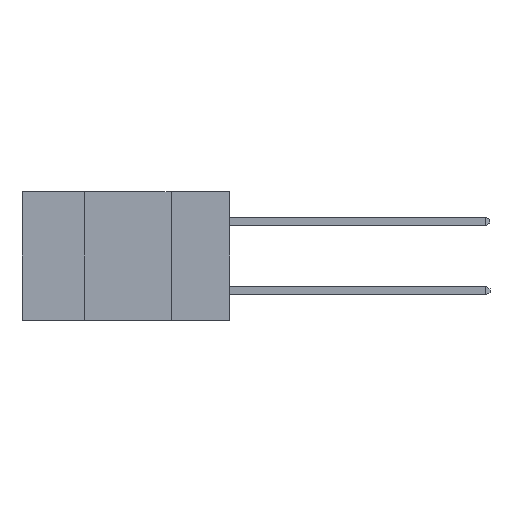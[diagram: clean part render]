
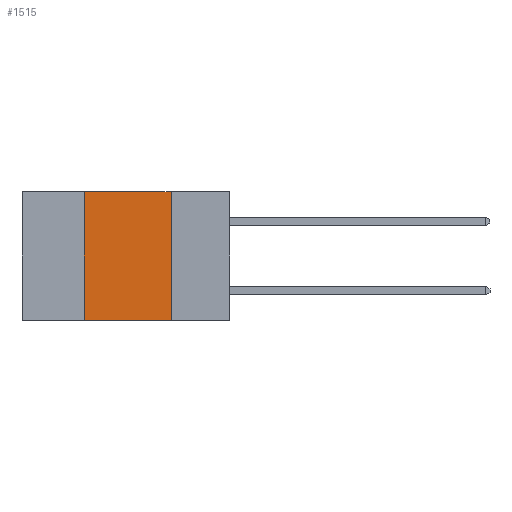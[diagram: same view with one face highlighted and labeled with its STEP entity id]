
A CAD part, left-side view. The second image highlights one B-rep face of the part: STEP entity #1515.
In plain terms, the highlighted planar face has unit normal (-1, 0, 0).
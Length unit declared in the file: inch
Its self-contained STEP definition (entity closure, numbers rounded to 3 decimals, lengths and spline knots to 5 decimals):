
#405 = VECTOR ( 'NONE', #3764, 39.37008 ) ;
#472 = CARTESIAN_POINT ( 'NONE',  ( 0., 0.6, 0. ) ) ;
#948 = LINE ( 'NONE', #8181, #2909 ) ;
#1068 = ORIENTED_EDGE ( 'NONE', *, *, #5798, .T. ) ;
#1515 = ADVANCED_FACE ( 'NONE', ( #8056 ), #9305, .F. ) ;
#2367 = CARTESIAN_POINT ( 'NONE',  ( 0., 0.42, 0. ) ) ;
#2909 = VECTOR ( 'NONE', #7818, 39.37008 ) ;
#3309 = CARTESIAN_POINT ( 'NONE',  ( 0., 0.42, -0.37 ) ) ;
#3413 = VERTEX_POINT ( 'NONE', #5740 ) ;
#3545 = ORIENTED_EDGE ( 'NONE', *, *, #8607, .F. ) ;
#3764 = DIRECTION ( 'NONE',  ( 0., 0., -1. ) ) ;
#3861 = CARTESIAN_POINT ( 'NONE',  ( 0., 0.17, 0. ) ) ;
#4043 = VERTEX_POINT ( 'NONE', #2367 ) ;
#4068 = VECTOR ( 'NONE', #9138, 39.37008 ) ;
#4483 = LINE ( 'NONE', #4726, #10520 ) ;
#4726 = CARTESIAN_POINT ( 'NONE',  ( 0., 0.6, 0. ) ) ;
#5127 = DIRECTION ( 'NONE',  ( 0., 0., -1. ) ) ;
#5740 = CARTESIAN_POINT ( 'NONE',  ( 0., 0.17, -0.37 ) ) ;
#5798 = EDGE_CURVE ( 'NONE', #10427, #3413, #948, .T. ) ;
#5991 = DIRECTION ( 'NONE',  ( 1., 0., 0. ) ) ;
#6003 = LINE ( 'NONE', #3309, #4068 ) ;
#6095 = VERTEX_POINT ( 'NONE', #3861 ) ;
#6387 = DIRECTION ( 'NONE',  ( 0., -1., 0. ) ) ;
#6858 = CARTESIAN_POINT ( 'NONE',  ( 0., 0.42, -0.37 ) ) ;
#6949 = EDGE_CURVE ( 'NONE', #10427, #4043, #6003, .T. ) ;
#7745 = ORIENTED_EDGE ( 'NONE', *, *, #6949, .F. ) ;
#7818 = DIRECTION ( 'NONE',  ( 0., -1., 0. ) ) ;
#8007 = ORIENTED_EDGE ( 'NONE', *, *, #9157, .F. ) ;
#8056 = FACE_OUTER_BOUND ( 'NONE', #10317, .T. ) ;
#8181 = CARTESIAN_POINT ( 'NONE',  ( 0., 0.6, -0.37 ) ) ;
#8589 = AXIS2_PLACEMENT_3D ( 'NONE', #472, #5991, #5127 ) ;
#8607 = EDGE_CURVE ( 'NONE', #4043, #6095, #4483, .T. ) ;
#8749 = CARTESIAN_POINT ( 'NONE',  ( 0., 0.17, -0.37 ) ) ;
#9138 = DIRECTION ( 'NONE',  ( 0., 0., 1. ) ) ;
#9157 = EDGE_CURVE ( 'NONE', #6095, #3413, #9257, .T. ) ;
#9257 = LINE ( 'NONE', #8749, #405 ) ;
#9305 = PLANE ( 'NONE',  #8589 ) ;
#10317 = EDGE_LOOP ( 'NONE', ( #8007, #3545, #7745, #1068 ) ) ;
#10427 = VERTEX_POINT ( 'NONE', #6858 ) ;
#10520 = VECTOR ( 'NONE', #6387, 39.37008 ) ;
